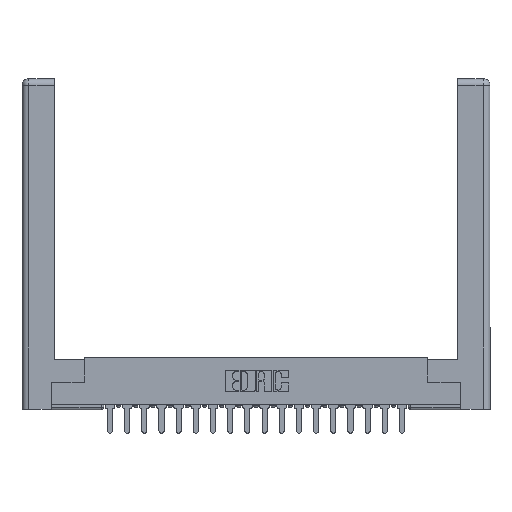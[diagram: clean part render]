
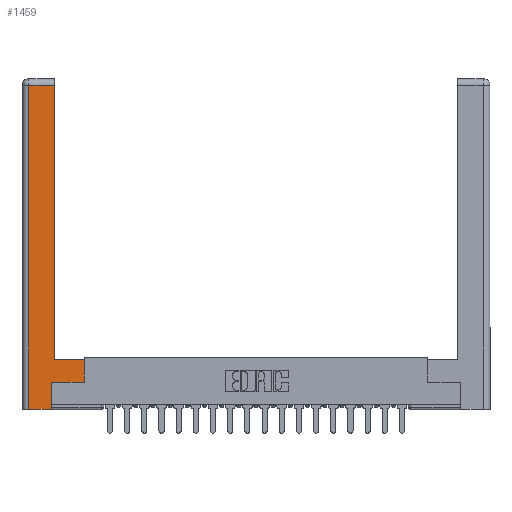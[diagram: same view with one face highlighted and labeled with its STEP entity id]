
A CAD part, top view. The second image highlights one B-rep face of the part: STEP entity #1459.
In plain terms, the highlighted planar face has unit normal (0, 0, 1).
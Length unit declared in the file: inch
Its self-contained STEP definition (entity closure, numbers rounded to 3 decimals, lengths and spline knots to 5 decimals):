
#555 = ORIENTED_EDGE ( 'NONE', *, *, #6511, .T. ) ;
#957 = CARTESIAN_POINT ( 'NONE',  ( 0.0615, 0., 0. ) ) ;
#1174 = DIRECTION ( 'NONE',  ( 0., 1., 0. ) ) ;
#1292 = DIRECTION ( 'NONE',  ( -1., 0., 0. ) ) ;
#1407 = CARTESIAN_POINT ( 'NONE',  ( 0.265, 0., 0. ) ) ;
#1459 = ADVANCED_FACE ( 'NONE', ( #10271 ), #4697, .F. ) ;
#1587 = VERTEX_POINT ( 'NONE', #16648 ) ;
#1970 = LINE ( 'NONE', #13191, #13862 ) ;
#2401 = VERTEX_POINT ( 'NONE', #19867 ) ;
#3007 = ORIENTED_EDGE ( 'NONE', *, *, #18397, .T. ) ;
#3530 = VECTOR ( 'NONE', #18534, 39.37008 ) ;
#3893 = CARTESIAN_POINT ( 'NONE',  ( 0.565, 0.245, 0. ) ) ;
#4445 = CARTESIAN_POINT ( 'NONE',  ( 0.565, 0.45, 0. ) ) ;
#4465 = VERTEX_POINT ( 'NONE', #7488 ) ;
#4672 = DIRECTION ( 'NONE',  ( 1., 0., 0. ) ) ;
#4691 = DIRECTION ( 'NONE',  ( 0., 1., 0. ) ) ;
#4697 = PLANE ( 'NONE',  #7809 ) ;
#5279 = ORIENTED_EDGE ( 'NONE', *, *, #13887, .T. ) ;
#5323 = CARTESIAN_POINT ( 'NONE',  ( 0.265, 0., 0. ) ) ;
#5453 = ORIENTED_EDGE ( 'NONE', *, *, #13396, .T. ) ;
#6242 = CARTESIAN_POINT ( 'NONE',  ( 0.265, 0.245, 0. ) ) ;
#6428 = EDGE_LOOP ( 'NONE', ( #555, #16286, #11071, #3007, #5279, #5453, #7573, #10180 ) ) ;
#6511 = EDGE_CURVE ( 'NONE', #1587, #4465, #1970, .T. ) ;
#6568 = VECTOR ( 'NONE', #18340, 39.37008 ) ;
#7144 = VERTEX_POINT ( 'NONE', #15782 ) ;
#7289 = CARTESIAN_POINT ( 'NONE',  ( 0.0615, 0., 0. ) ) ;
#7488 = CARTESIAN_POINT ( 'NONE',  ( 0.295, 2.94, 0. ) ) ;
#7573 = ORIENTED_EDGE ( 'NONE', *, *, #13685, .T. ) ;
#7809 = AXIS2_PLACEMENT_3D ( 'NONE', #20710, #10967, #1292 ) ;
#7874 = DIRECTION ( 'NONE',  ( -1., 0., 0. ) ) ;
#8106 = LINE ( 'NONE', #3893, #3530 ) ;
#8856 = VECTOR ( 'NONE', #1174, 39.37008 ) ;
#9121 = LINE ( 'NONE', #19043, #12152 ) ;
#9798 = DIRECTION ( 'NONE',  ( 0., 1., 0. ) ) ;
#10180 = ORIENTED_EDGE ( 'NONE', *, *, #14364, .T. ) ;
#10271 = FACE_OUTER_BOUND ( 'NONE', #6428, .T. ) ;
#10346 = VECTOR ( 'NONE', #4691, 39.37008 ) ;
#10696 = DIRECTION ( 'NONE',  ( 0., -1., 0. ) ) ;
#10967 = DIRECTION ( 'NONE',  ( 0., 0., -1. ) ) ;
#11071 = ORIENTED_EDGE ( 'NONE', *, *, #20883, .T. ) ;
#11419 = VECTOR ( 'NONE', #4672, 39.37008 ) ;
#11557 = CARTESIAN_POINT ( 'NONE',  ( 0.0615, 2.94, 0. ) ) ;
#11880 = LINE ( 'NONE', #6242, #10346 ) ;
#12152 = VECTOR ( 'NONE', #7874, 39.37008 ) ;
#12589 = VECTOR ( 'NONE', #10696, 39.37008 ) ;
#13153 = LINE ( 'NONE', #4445, #8856 ) ;
#13191 = CARTESIAN_POINT ( 'NONE',  ( 0.295, 3., 0. ) ) ;
#13224 = EDGE_CURVE ( 'NONE', #4465, #16822, #9121, .T. ) ;
#13396 = EDGE_CURVE ( 'NONE', #7144, #16258, #8106, .T. ) ;
#13685 = EDGE_CURVE ( 'NONE', #16258, #2401, #13153, .T. ) ;
#13862 = VECTOR ( 'NONE', #9798, 39.37008 ) ;
#13887 = EDGE_CURVE ( 'NONE', #17536, #7144, #11880, .T. ) ;
#14364 = EDGE_CURVE ( 'NONE', #2401, #1587, #14696, .T. ) ;
#14696 = LINE ( 'NONE', #14994, #6568 ) ;
#14994 = CARTESIAN_POINT ( 'NONE',  ( 0.295, 0.45, 0. ) ) ;
#15138 = VERTEX_POINT ( 'NONE', #7289 ) ;
#15490 = LINE ( 'NONE', #1407, #11419 ) ;
#15782 = CARTESIAN_POINT ( 'NONE',  ( 0.265, 0.245, 0. ) ) ;
#15903 = LINE ( 'NONE', #957, #12589 ) ;
#16258 = VERTEX_POINT ( 'NONE', #19921 ) ;
#16286 = ORIENTED_EDGE ( 'NONE', *, *, #13224, .T. ) ;
#16648 = CARTESIAN_POINT ( 'NONE',  ( 0.295, 0.45, 0. ) ) ;
#16822 = VERTEX_POINT ( 'NONE', #11557 ) ;
#17536 = VERTEX_POINT ( 'NONE', #5323 ) ;
#18340 = DIRECTION ( 'NONE',  ( -1., 0., 0. ) ) ;
#18397 = EDGE_CURVE ( 'NONE', #15138, #17536, #15490, .T. ) ;
#18534 = DIRECTION ( 'NONE',  ( 1., 0., 0. ) ) ;
#19043 = CARTESIAN_POINT ( 'NONE',  ( 0.0615, 2.94, 0. ) ) ;
#19867 = CARTESIAN_POINT ( 'NONE',  ( 0.565, 0.45, 0. ) ) ;
#19921 = CARTESIAN_POINT ( 'NONE',  ( 0.565, 0.245, 0. ) ) ;
#20710 = CARTESIAN_POINT ( 'NONE',  ( 0., 0., 0. ) ) ;
#20883 = EDGE_CURVE ( 'NONE', #16822, #15138, #15903, .T. ) ;
